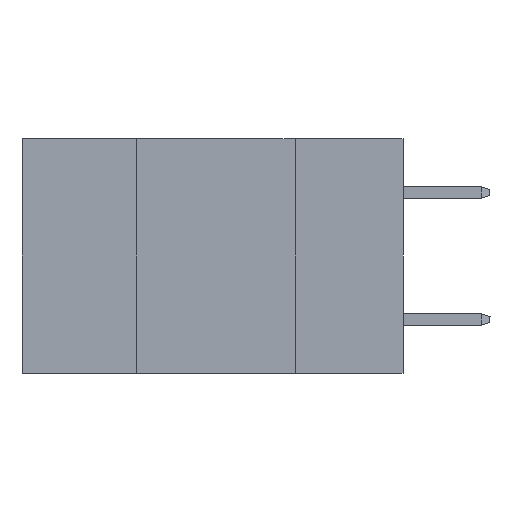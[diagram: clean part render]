
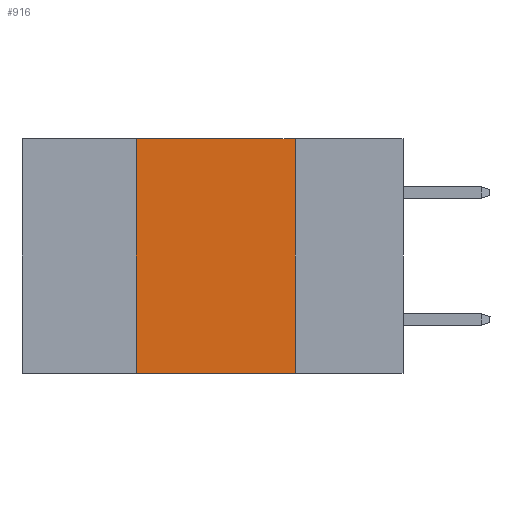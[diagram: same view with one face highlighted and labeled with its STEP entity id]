
A CAD part, left-side view. The second image highlights one B-rep face of the part: STEP entity #916.
In plain terms, the highlighted planar face has unit normal (-1, 0, 0).
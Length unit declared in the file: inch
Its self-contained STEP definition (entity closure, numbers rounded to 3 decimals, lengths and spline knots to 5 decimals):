
#203 = ORIENTED_EDGE ( 'NONE', *, *, #18001, .F. ) ;
#332 = EDGE_CURVE ( 'NONE', #4235, #10759, #3894, .T. ) ;
#388 = EDGE_LOOP ( 'NONE', ( #10245, #2535, #203, #11033 ) ) ;
#553 = FACE_OUTER_BOUND ( 'NONE', #388, .T. ) ;
#916 = ADVANCED_FACE ( 'NONE', ( #553 ), #2252, .F. ) ;
#1460 = DIRECTION ( 'NONE',  ( 0., 0., 1. ) ) ;
#1969 = DIRECTION ( 'NONE',  ( 0., -1., 0. ) ) ;
#2252 = PLANE ( 'NONE',  #11023 ) ;
#2535 = ORIENTED_EDGE ( 'NONE', *, *, #9481, .F. ) ;
#3894 = LINE ( 'NONE', #9923, #6568 ) ;
#4068 = LINE ( 'NONE', #5948, #14088 ) ;
#4235 = VERTEX_POINT ( 'NONE', #15303 ) ;
#5948 = CARTESIAN_POINT ( 'NONE',  ( 0., 0.17, 0. ) ) ;
#6568 = VECTOR ( 'NONE', #18801, 39.37008 ) ;
#6600 = DIRECTION ( 'NONE',  ( 0., 0., -1. ) ) ;
#6628 = CARTESIAN_POINT ( 'NONE',  ( 0., 0.42, 0. ) ) ;
#8044 = VECTOR ( 'NONE', #1969, 39.37008 ) ;
#8612 = DIRECTION ( 'NONE',  ( 0., 0., -1. ) ) ;
#9481 = EDGE_CURVE ( 'NONE', #12039, #18413, #11160, .T. ) ;
#9923 = CARTESIAN_POINT ( 'NONE',  ( 0., 0.6, -0.37 ) ) ;
#10245 = ORIENTED_EDGE ( 'NONE', *, *, #13507, .F. ) ;
#10759 = VERTEX_POINT ( 'NONE', #10880 ) ;
#10880 = CARTESIAN_POINT ( 'NONE',  ( 0., 0.17, -0.37 ) ) ;
#11023 = AXIS2_PLACEMENT_3D ( 'NONE', #11158, #15691, #6600 ) ;
#11033 = ORIENTED_EDGE ( 'NONE', *, *, #332, .T. ) ;
#11158 = CARTESIAN_POINT ( 'NONE',  ( 0., 0.6, 0. ) ) ;
#11160 = LINE ( 'NONE', #17373, #8044 ) ;
#12039 = VERTEX_POINT ( 'NONE', #6628 ) ;
#13507 = EDGE_CURVE ( 'NONE', #18413, #10759, #4068, .T. ) ;
#13739 = CARTESIAN_POINT ( 'NONE',  ( 0., 0.17, 0. ) ) ;
#14088 = VECTOR ( 'NONE', #8612, 39.37008 ) ;
#14994 = CARTESIAN_POINT ( 'NONE',  ( 0., 0.42, 0. ) ) ;
#15303 = CARTESIAN_POINT ( 'NONE',  ( 0., 0.42, -0.37 ) ) ;
#15691 = DIRECTION ( 'NONE',  ( 1., 0., 0. ) ) ;
#16679 = LINE ( 'NONE', #14994, #17736 ) ;
#17373 = CARTESIAN_POINT ( 'NONE',  ( 0., 0.6, 0. ) ) ;
#17736 = VECTOR ( 'NONE', #1460, 39.37008 ) ;
#18001 = EDGE_CURVE ( 'NONE', #4235, #12039, #16679, .T. ) ;
#18413 = VERTEX_POINT ( 'NONE', #13739 ) ;
#18801 = DIRECTION ( 'NONE',  ( 0., -1., 0. ) ) ;
